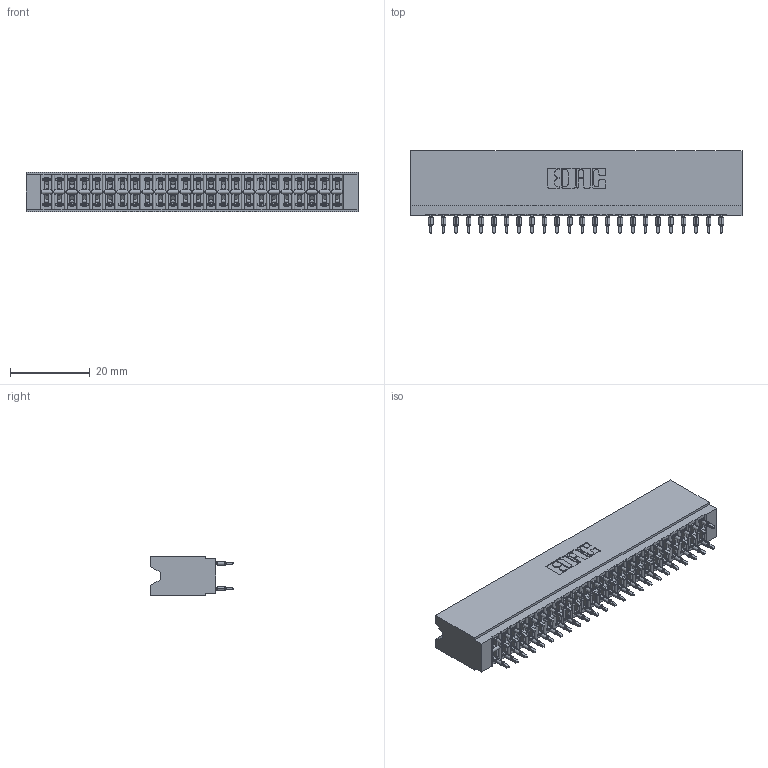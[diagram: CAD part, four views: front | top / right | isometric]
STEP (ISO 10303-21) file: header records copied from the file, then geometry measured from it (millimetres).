
FILE_DESCRIPTION (( 'STEP AP203' ), '1' );
FILE_NAME ('746-048-560-206.STEP', '2020-09-17T01:46:08', ( '' ), ( '' ), 'SwSTEP 2.0', 'SolidWorks 2020', '' );
FILE_SCHEMA (( 'CONFIG_CONTROL_DESIGN' ));
Length unit declared in the file: inch
Products named in the file (3): 746-048-560-206; 746-292-001_560; 746 Part_.515 Slot Depth - 06
Assembly tree (49 placements, depth 2):
  746-048-560-206
    746 Part_.515 Slot Depth - 06
    746-292-001_560  x48
Bounding box: 83.44 x 20.82 x 9.91 mm (x, y, z)
Volume: 9220.1 mm3; surface area: 15364.6 mm2
Topology: 49 solids, 49 shells, 4634 faces, 12889 edges, 8263 vertices
Faces by surface type: plane 2312, cylinder 1074, bspline 960, torus 288
Entity records: 39790 total; most frequent: CARTESIAN_POINT 8062, ORIENTED_EDGE 6790, DIRECTION 5707, EDGE_CURVE 3395, VECTOR 2963, LINE 2963, VERTEX_POINT 2247, AXIS2_PLACEMENT_3D 1372
